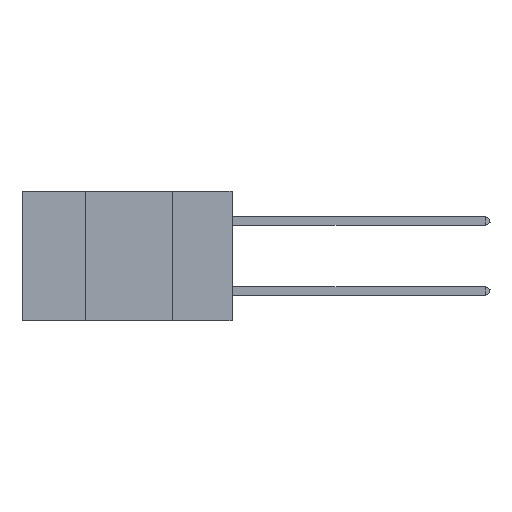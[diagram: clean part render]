
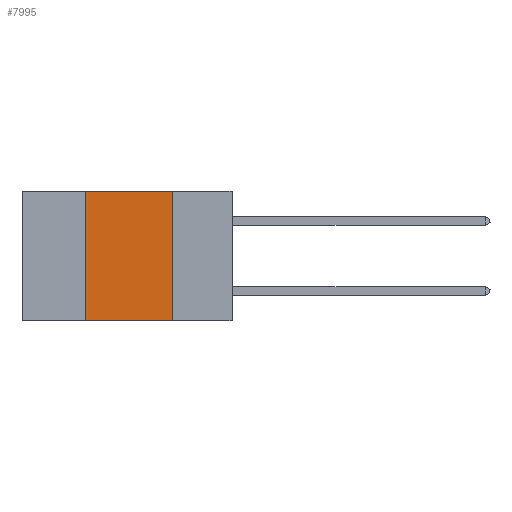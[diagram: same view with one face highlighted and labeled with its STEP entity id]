
A CAD part, left-side view. The second image highlights one B-rep face of the part: STEP entity #7995.
In plain terms, the highlighted planar face has unit normal (-1, 0, 0).
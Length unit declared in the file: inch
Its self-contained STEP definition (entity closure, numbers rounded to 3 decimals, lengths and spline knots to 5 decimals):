
#282 = EDGE_CURVE ( 'NONE', #17939, #41150, #40682, .T. ) ;
#629 = LINE ( 'NONE', #10839, #4735 ) ;
#785 = CARTESIAN_POINT ( 'NONE',  ( 0., 0.17, -0.37 ) ) ;
#1154 = VECTOR ( 'NONE', #21135, 39.37008 ) ;
#1852 = CARTESIAN_POINT ( 'NONE',  ( 0., 0.6, 0. ) ) ;
#4258 = DIRECTION ( 'NONE',  ( 0., -1., 0. ) ) ;
#4735 = VECTOR ( 'NONE', #40943, 39.37008 ) ;
#7995 = ADVANCED_FACE ( 'NONE', ( #42029 ), #46742, .F. ) ;
#8449 = CARTESIAN_POINT ( 'NONE',  ( 0., 0.42, 0. ) ) ;
#10335 = ORIENTED_EDGE ( 'NONE', *, *, #44749, .F. ) ;
#10839 = CARTESIAN_POINT ( 'NONE',  ( 0., 0.6, 0. ) ) ;
#11148 = LINE ( 'NONE', #16578, #1154 ) ;
#11689 = VERTEX_POINT ( 'NONE', #22699 ) ;
#12587 = EDGE_CURVE ( 'NONE', #11689, #41150, #11148, .T. ) ;
#12595 = VECTOR ( 'NONE', #4258, 39.37008 ) ;
#13858 = VECTOR ( 'NONE', #34624, 39.37008 ) ;
#14235 = EDGE_CURVE ( 'NONE', #17939, #47148, #34384, .T. ) ;
#16578 = CARTESIAN_POINT ( 'NONE',  ( 0., 0.17, 0. ) ) ;
#16776 = AXIS2_PLACEMENT_3D ( 'NONE', #1852, #20672, #31630 ) ;
#17939 = VERTEX_POINT ( 'NONE', #20166 ) ;
#20166 = CARTESIAN_POINT ( 'NONE',  ( 0., 0.42, -0.37 ) ) ;
#20672 = DIRECTION ( 'NONE',  ( 1., 0., 0. ) ) ;
#21135 = DIRECTION ( 'NONE',  ( 0., 0., -1. ) ) ;
#22699 = CARTESIAN_POINT ( 'NONE',  ( 0., 0.17, 0. ) ) ;
#27583 = CARTESIAN_POINT ( 'NONE',  ( 0., 0.42, 0. ) ) ;
#30979 = ORIENTED_EDGE ( 'NONE', *, *, #282, .T. ) ;
#31630 = DIRECTION ( 'NONE',  ( 0., 0., -1. ) ) ;
#34384 = LINE ( 'NONE', #8449, #13858 ) ;
#34624 = DIRECTION ( 'NONE',  ( 0., 0., 1. ) ) ;
#39185 = CARTESIAN_POINT ( 'NONE',  ( 0., 0.6, -0.37 ) ) ;
#39322 = ORIENTED_EDGE ( 'NONE', *, *, #14235, .F. ) ;
#40682 = LINE ( 'NONE', #39185, #12595 ) ;
#40943 = DIRECTION ( 'NONE',  ( 0., -1., 0. ) ) ;
#41150 = VERTEX_POINT ( 'NONE', #785 ) ;
#41224 = ORIENTED_EDGE ( 'NONE', *, *, #12587, .F. ) ;
#42029 = FACE_OUTER_BOUND ( 'NONE', #47471, .T. ) ;
#44749 = EDGE_CURVE ( 'NONE', #47148, #11689, #629, .T. ) ;
#46742 = PLANE ( 'NONE',  #16776 ) ;
#47148 = VERTEX_POINT ( 'NONE', #27583 ) ;
#47471 = EDGE_LOOP ( 'NONE', ( #41224, #10335, #39322, #30979 ) ) ;
